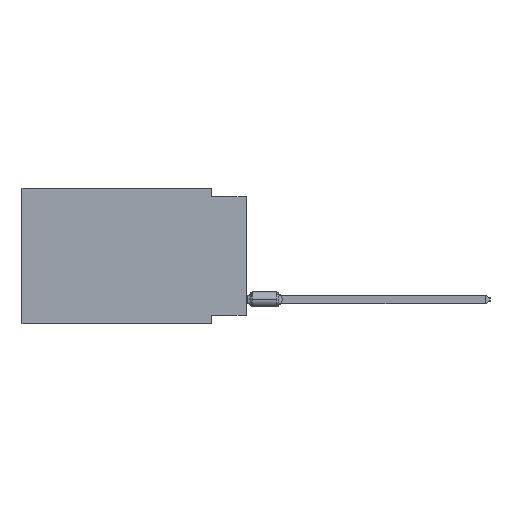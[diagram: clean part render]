
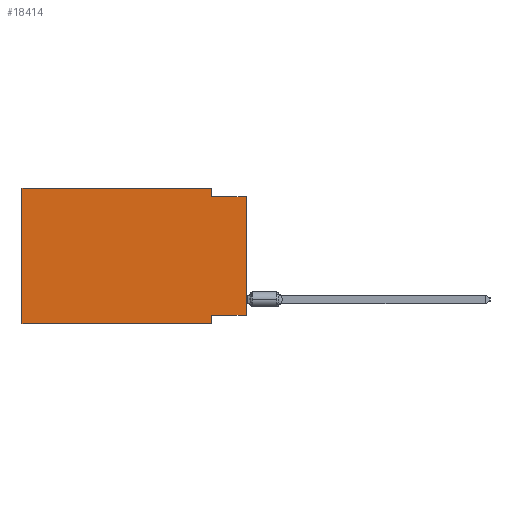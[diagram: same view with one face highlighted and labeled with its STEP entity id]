
A CAD part, left-side view. The second image highlights one B-rep face of the part: STEP entity #18414.
In plain terms, the highlighted planar face has unit normal (-1, 0, 0).
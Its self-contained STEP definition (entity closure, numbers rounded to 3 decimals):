
#35 = VECTOR ( 'NONE', #45797, 1000. ) ;
#2634 = LINE ( 'NONE', #7763, #45410 ) ;
#3930 = VERTEX_POINT ( 'NONE', #70525 ) ;
#5250 = CARTESIAN_POINT ( 'NONE',  ( 0., 16.383, -9.906 ) ) ;
#5648 = EDGE_CURVE ( 'NONE', #12522, #61914, #13522, .T. ) ;
#6132 = VERTEX_POINT ( 'NONE', #62091 ) ;
#6403 = ORIENTED_EDGE ( 'NONE', *, *, #28093, .F. ) ;
#7763 = CARTESIAN_POINT ( 'NONE',  ( 0., 0., -9.271 ) ) ;
#8520 = LINE ( 'NONE', #33591, #26418 ) ;
#9829 = ORIENTED_EDGE ( 'NONE', *, *, #74819, .T. ) ;
#9839 = DIRECTION ( 'NONE',  ( 0., 0., 1. ) ) ;
#12522 = VERTEX_POINT ( 'NONE', #61386 ) ;
#13522 = LINE ( 'NONE', #78093, #35 ) ;
#14437 = EDGE_CURVE ( 'NONE', #68417, #80427, #38687, .T. ) ;
#14444 = CARTESIAN_POINT ( 'NONE',  ( 0., 0., 0. ) ) ;
#15786 = CARTESIAN_POINT ( 'NONE',  ( 0., 16.383, 0. ) ) ;
#15973 = LINE ( 'NONE', #74180, #49176 ) ;
#18183 = LINE ( 'NONE', #57692, #32557 ) ;
#18414 = ADVANCED_FACE ( 'NONE', ( #78394 ), #66079, .F. ) ;
#20200 = CARTESIAN_POINT ( 'NONE',  ( 0., 16.383, 0. ) ) ;
#25066 = CARTESIAN_POINT ( 'NONE',  ( 0., 2.54, -9.271 ) ) ;
#26249 = EDGE_CURVE ( 'NONE', #68417, #12522, #48055, .T. ) ;
#26418 = VECTOR ( 'NONE', #34423, 1000. ) ;
#27012 = EDGE_LOOP ( 'NONE', ( #9829, #6403, #34889, #58292, #48285, #51046, #64312, #75606 ) ) ;
#28093 = EDGE_CURVE ( 'NONE', #6132, #61262, #15973, .T. ) ;
#31706 = CARTESIAN_POINT ( 'NONE',  ( 0., 0., -0.635 ) ) ;
#32557 = VECTOR ( 'NONE', #62375, 1000. ) ;
#33591 = CARTESIAN_POINT ( 'NONE',  ( 0., 2.54, -9.906 ) ) ;
#34423 = DIRECTION ( 'NONE',  ( 0., 0., -1. ) ) ;
#34889 = ORIENTED_EDGE ( 'NONE', *, *, #39490, .F. ) ;
#36660 = CARTESIAN_POINT ( 'NONE',  ( 0., 2.54, -9.906 ) ) ;
#38687 = LINE ( 'NONE', #64629, #66275 ) ;
#39490 = EDGE_CURVE ( 'NONE', #61914, #6132, #18183, .T. ) ;
#41264 = DIRECTION ( 'NONE',  ( 0., 1., 0. ) ) ;
#41876 = DIRECTION ( 'NONE',  ( 0., -1., 0. ) ) ;
#45141 = AXIS2_PLACEMENT_3D ( 'NONE', #20200, #46104, #72040 ) ;
#45410 = VECTOR ( 'NONE', #41264, 1000. ) ;
#45797 = DIRECTION ( 'NONE',  ( 0., -1., 0. ) ) ;
#46104 = DIRECTION ( 'NONE',  ( 1., 0., 0. ) ) ;
#46331 = VECTOR ( 'NONE', #47957, 1000. ) ;
#47957 = DIRECTION ( 'NONE',  ( 0., 0., 1. ) ) ;
#48055 = LINE ( 'NONE', #15786, #49986 ) ;
#48285 = ORIENTED_EDGE ( 'NONE', *, *, #26249, .F. ) ;
#49176 = VECTOR ( 'NONE', #41876, 1000. ) ;
#49986 = VECTOR ( 'NONE', #9839, 1000. ) ;
#51046 = ORIENTED_EDGE ( 'NONE', *, *, #14437, .T. ) ;
#51073 = EDGE_CURVE ( 'NONE', #53326, #80427, #8520, .T. ) ;
#53326 = VERTEX_POINT ( 'NONE', #25066 ) ;
#57692 = CARTESIAN_POINT ( 'NONE',  ( 0., 2.54, 0. ) ) ;
#58292 = ORIENTED_EDGE ( 'NONE', *, *, #5648, .F. ) ;
#61262 = VERTEX_POINT ( 'NONE', #31706 ) ;
#61386 = CARTESIAN_POINT ( 'NONE',  ( 0., 16.383, 0. ) ) ;
#61914 = VERTEX_POINT ( 'NONE', #81636 ) ;
#62091 = CARTESIAN_POINT ( 'NONE',  ( 0., 2.54, -0.635 ) ) ;
#62375 = DIRECTION ( 'NONE',  ( 0., 0., -1. ) ) ;
#64312 = ORIENTED_EDGE ( 'NONE', *, *, #51073, .F. ) ;
#64629 = CARTESIAN_POINT ( 'NONE',  ( 0., 16.383, -9.906 ) ) ;
#66079 = PLANE ( 'NONE',  #45141 ) ;
#66275 = VECTOR ( 'NONE', #77776, 1000. ) ;
#68417 = VERTEX_POINT ( 'NONE', #5250 ) ;
#70525 = CARTESIAN_POINT ( 'NONE',  ( 0., 0., -9.271 ) ) ;
#72040 = DIRECTION ( 'NONE',  ( 0., 0., -1. ) ) ;
#74180 = CARTESIAN_POINT ( 'NONE',  ( 0., 0., -0.635 ) ) ;
#74819 = EDGE_CURVE ( 'NONE', #3930, #61262, #80676, .T. ) ;
#75606 = ORIENTED_EDGE ( 'NONE', *, *, #80638, .F. ) ;
#77776 = DIRECTION ( 'NONE',  ( 0., -1., 0. ) ) ;
#78093 = CARTESIAN_POINT ( 'NONE',  ( 0., 16.383, 0. ) ) ;
#78394 = FACE_OUTER_BOUND ( 'NONE', #27012, .T. ) ;
#80427 = VERTEX_POINT ( 'NONE', #36660 ) ;
#80638 = EDGE_CURVE ( 'NONE', #3930, #53326, #2634, .T. ) ;
#80676 = LINE ( 'NONE', #14444, #46331 ) ;
#81636 = CARTESIAN_POINT ( 'NONE',  ( 0., 2.54, 0. ) ) ;
